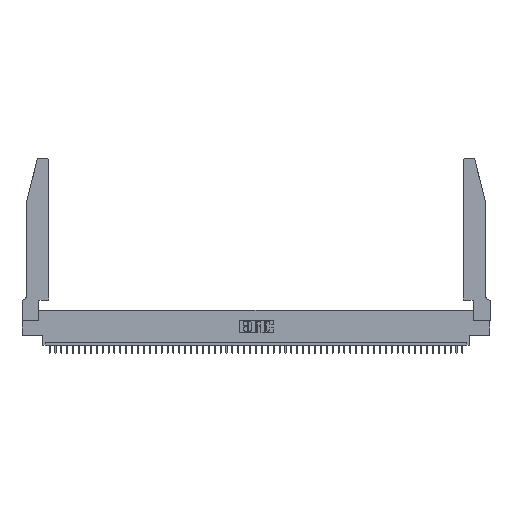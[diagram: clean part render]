
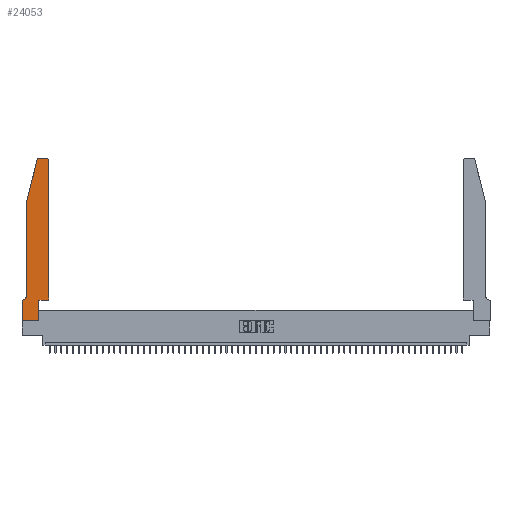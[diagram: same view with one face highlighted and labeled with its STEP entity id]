
A CAD part, top view. The second image highlights one B-rep face of the part: STEP entity #24053.
In plain terms, the highlighted planar face has unit normal (0, 0, 1).
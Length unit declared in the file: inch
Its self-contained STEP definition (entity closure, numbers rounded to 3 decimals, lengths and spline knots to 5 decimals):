
#374 = CARTESIAN_POINT ( 'NONE',  ( 0.0755, 0.42, 0.37 ) ) ;
#709 = DIRECTION ( 'NONE',  ( -0.239, -0.971, 0. ) ) ;
#1486 = LINE ( 'NONE', #38947, #9983 ) ;
#1909 = VERTEX_POINT ( 'NONE', #8159 ) ;
#2118 = ORIENTED_EDGE ( 'NONE', *, *, #50013, .T. ) ;
#2228 = VERTEX_POINT ( 'NONE', #45531 ) ;
#2570 = ORIENTED_EDGE ( 'NONE', *, *, #20445, .T. ) ;
#3047 = VERTEX_POINT ( 'NONE', #4333 ) ;
#4051 = ORIENTED_EDGE ( 'NONE', *, *, #53648, .T. ) ;
#4287 = DIRECTION ( 'NONE',  ( 0., 1., 0. ) ) ;
#4333 = CARTESIAN_POINT ( 'NONE',  ( 0., 0.35, 0.37 ) ) ;
#5631 = VECTOR ( 'NONE', #709, 39.37008 ) ;
#5774 = CARTESIAN_POINT ( 'NONE',  ( 0.2605, 2.75, 0.37 ) ) ;
#6054 = DIRECTION ( 'NONE',  ( -1., 0., 0. ) ) ;
#6816 = DIRECTION ( 'NONE',  ( 1., 0., 0. ) ) ;
#6871 = VECTOR ( 'NONE', #10470, 39.37008 ) ;
#7607 = EDGE_CURVE ( 'NONE', #2228, #43371, #19520, .T. ) ;
#8022 = LINE ( 'NONE', #45796, #50264 ) ;
#8159 = CARTESIAN_POINT ( 'NONE',  ( 0.0055, 0.35, 0.37 ) ) ;
#8523 = ORIENTED_EDGE ( 'NONE', *, *, #7607, .T. ) ;
#8667 = CARTESIAN_POINT ( 'NONE',  ( 0.4505, 0.35, 0.37 ) ) ;
#9293 = DIRECTION ( 'NONE',  ( 0., 1., 0. ) ) ;
#9983 = VECTOR ( 'NONE', #43380, 39.37008 ) ;
#10470 = DIRECTION ( 'NONE',  ( -1., 0., 0. ) ) ;
#11148 = ORIENTED_EDGE ( 'NONE', *, *, #52058, .T. ) ;
#11733 = CARTESIAN_POINT ( 'NONE',  ( 0.2865, 0., 0.37 ) ) ;
#11804 = VERTEX_POINT ( 'NONE', #47135 ) ;
#12506 = DIRECTION ( 'NONE',  ( 0., 0., 1. ) ) ;
#12649 = VECTOR ( 'NONE', #9293, 39.37008 ) ;
#14862 = VECTOR ( 'NONE', #6054, 39.37008 ) ;
#15074 = CARTESIAN_POINT ( 'NONE',  ( 0.4205, 2.72, 0.37 ) ) ;
#15287 = VERTEX_POINT ( 'NONE', #25634 ) ;
#15995 = EDGE_CURVE ( 'NONE', #19912, #33232, #35617, .T. ) ;
#17201 = LINE ( 'NONE', #8667, #51788 ) ;
#17735 = DIRECTION ( 'NONE',  ( 0., 0., -1. ) ) ;
#18659 = FACE_OUTER_BOUND ( 'NONE', #48186, .T. ) ;
#19077 = DIRECTION ( 'NONE',  ( 1., 0., 0. ) ) ;
#19520 = LINE ( 'NONE', #5774, #14862 ) ;
#19783 = VERTEX_POINT ( 'NONE', #374 ) ;
#19912 = VERTEX_POINT ( 'NONE', #42309 ) ;
#20445 = EDGE_CURVE ( 'NONE', #15287, #2228, #33027, .T. ) ;
#20792 = DIRECTION ( 'NONE',  ( -1., 0., 0. ) ) ;
#21692 = LINE ( 'NONE', #39030, #12649 ) ;
#22413 = CIRCLE ( 'NONE', #53224, 0.03 ) ;
#22979 = ORIENTED_EDGE ( 'NONE', *, *, #15995, .T. ) ;
#23360 = ORIENTED_EDGE ( 'NONE', *, *, #31516, .T. ) ;
#23477 = EDGE_CURVE ( 'NONE', #24187, #41237, #29788, .T. ) ;
#23622 = AXIS2_PLACEMENT_3D ( 'NONE', #47252, #17735, #20792 ) ;
#24053 = ADVANCED_FACE ( 'NONE', ( #18659 ), #47908, .T. ) ;
#24187 = VERTEX_POINT ( 'NONE', #36546 ) ;
#25634 = CARTESIAN_POINT ( 'NONE',  ( 0.4505, 2.72, 0.37 ) ) ;
#25995 = EDGE_CURVE ( 'NONE', #19783, #1909, #52679, .T. ) ;
#26037 = EDGE_CURVE ( 'NONE', #33232, #15287, #17201, .T. ) ;
#26214 = CARTESIAN_POINT ( 'NONE',  ( 0., 0., 0.37 ) ) ;
#26332 = CARTESIAN_POINT ( 'NONE',  ( 0.0755, 2., 0.37 ) ) ;
#27016 = LINE ( 'NONE', #39678, #6871 ) ;
#29335 = DIRECTION ( 'NONE',  ( 1., 0., 0. ) ) ;
#29788 = LINE ( 'NONE', #26214, #49872 ) ;
#30865 = CARTESIAN_POINT ( 'NONE',  ( 0.25487, 2.72718, 0.37 ) ) ;
#31516 = EDGE_CURVE ( 'NONE', #1909, #3047, #27016, .T. ) ;
#31901 = DIRECTION ( 'NONE',  ( 1., 0., 0. ) ) ;
#33027 = CIRCLE ( 'NONE', #37417, 0.03 ) ;
#33232 = VERTEX_POINT ( 'NONE', #48169 ) ;
#34282 = ORIENTED_EDGE ( 'NONE', *, *, #25995, .T. ) ;
#34937 = DIRECTION ( 'NONE',  ( 0., 0., 1. ) ) ;
#34985 = ORIENTED_EDGE ( 'NONE', *, *, #39801, .T. ) ;
#35617 = LINE ( 'NONE', #40019, #45289 ) ;
#35975 = EDGE_CURVE ( 'NONE', #11804, #19783, #8022, .T. ) ;
#36007 = DIRECTION ( 'NONE',  ( 0., 0., 1. ) ) ;
#36546 = CARTESIAN_POINT ( 'NONE',  ( 0., 0., 0.37 ) ) ;
#37417 = AXIS2_PLACEMENT_3D ( 'NONE', #15074, #36007, #31901 ) ;
#37953 = ORIENTED_EDGE ( 'NONE', *, *, #26037, .T. ) ;
#38947 = CARTESIAN_POINT ( 'NONE',  ( 0., 0., 0.37 ) ) ;
#39030 = CARTESIAN_POINT ( 'NONE',  ( 0.2865, 0.35, 0.37 ) ) ;
#39339 = CARTESIAN_POINT ( 'NONE',  ( 0., 0.35, 0.37 ) ) ;
#39678 = CARTESIAN_POINT ( 'NONE',  ( 0.0755, 0.35, 0.37 ) ) ;
#39801 = EDGE_CURVE ( 'NONE', #41237, #19912, #21692, .T. ) ;
#40019 = CARTESIAN_POINT ( 'NONE',  ( 0.4505, 0.35, 0.37 ) ) ;
#40563 = VERTEX_POINT ( 'NONE', #30865 ) ;
#41237 = VERTEX_POINT ( 'NONE', #11733 ) ;
#42308 = CARTESIAN_POINT ( 'NONE',  ( 0.284, 2.72, 0.37 ) ) ;
#42309 = CARTESIAN_POINT ( 'NONE',  ( 0.2865, 0.35, 0.37 ) ) ;
#42791 = CARTESIAN_POINT ( 'NONE',  ( 0.284, 2.75, 0.37 ) ) ;
#43371 = VERTEX_POINT ( 'NONE', #42791 ) ;
#43380 = DIRECTION ( 'NONE',  ( 0., -1., 0. ) ) ;
#45289 = VECTOR ( 'NONE', #19077, 39.37008 ) ;
#45531 = CARTESIAN_POINT ( 'NONE',  ( 0.4205, 2.75, 0.37 ) ) ;
#45796 = CARTESIAN_POINT ( 'NONE',  ( 0.0755, 2., 0.37 ) ) ;
#46026 = ORIENTED_EDGE ( 'NONE', *, *, #35975, .T. ) ;
#47135 = CARTESIAN_POINT ( 'NONE',  ( 0.0755, 2., 0.37 ) ) ;
#47252 = CARTESIAN_POINT ( 'NONE',  ( 0.0055, 0.42, 0.37 ) ) ;
#47908 = PLANE ( 'NONE',  #48982 ) ;
#48169 = CARTESIAN_POINT ( 'NONE',  ( 0.4505, 0.35, 0.37 ) ) ;
#48186 = EDGE_LOOP ( 'NONE', ( #8523, #4051, #11148, #46026, #34282, #23360, #2118, #52203, #34985, #22979, #37953, #2570 ) ) ;
#48982 = AXIS2_PLACEMENT_3D ( 'NONE', #39339, #34937, #6816 ) ;
#49872 = VECTOR ( 'NONE', #51287, 39.37008 ) ;
#50013 = EDGE_CURVE ( 'NONE', #3047, #24187, #1486, .T. ) ;
#50264 = VECTOR ( 'NONE', #54358, 39.37008 ) ;
#51148 = LINE ( 'NONE', #26332, #5631 ) ;
#51287 = DIRECTION ( 'NONE',  ( 1., 0., 0. ) ) ;
#51788 = VECTOR ( 'NONE', #4287, 39.37008 ) ;
#52058 = EDGE_CURVE ( 'NONE', #40563, #11804, #51148, .T. ) ;
#52203 = ORIENTED_EDGE ( 'NONE', *, *, #23477, .T. ) ;
#52679 = CIRCLE ( 'NONE', #23622, 0.07 ) ;
#53224 = AXIS2_PLACEMENT_3D ( 'NONE', #42308, #12506, #29335 ) ;
#53648 = EDGE_CURVE ( 'NONE', #43371, #40563, #22413, .T. ) ;
#54358 = DIRECTION ( 'NONE',  ( 0., -1., 0. ) ) ;
